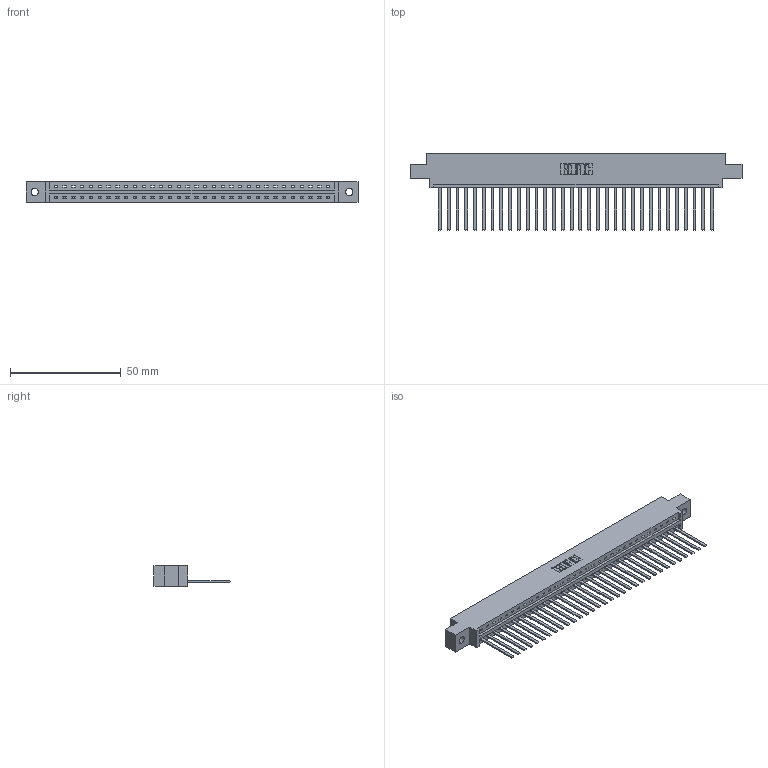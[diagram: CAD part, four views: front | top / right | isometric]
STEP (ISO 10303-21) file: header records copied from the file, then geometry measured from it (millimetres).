
FILE_DESCRIPTION (( 'STEP AP203' ), '1' );
FILE_NAME ('337-032-544-602.STEP', '2019-10-01T03:38:25', ( '' ), ( '' ), 'SwSTEP 2.0', 'SolidWorks 2016', '' );
FILE_SCHEMA (( 'CONFIG_CONTROL_DESIGN' ));
Length unit declared in the file: inch
Products named in the file (3): 337 Part_0.170 Offset - 0.128 Dia; 337-032-544-602; 345-292-001_345-293-144
Assembly tree (33 placements, depth 2):
  337-032-544-602
    337 Part_0.170 Offset - 0.128 Dia
    345-292-001_345-293-144  x32
Bounding box: 149.81 x 34.3 x 9.4 mm (x, y, z)
Volume: 15661.4 mm3; surface area: 17174 mm2
Topology: 33 solids, 33 shells, 1910 faces, 5763 edges, 3798 vertices
Faces by surface type: plane 1418, cylinder 492
Entity records: 25031 total; most frequent: CARTESIAN_POINT 4366, ORIENTED_EDGE 4334, DIRECTION 3691, EDGE_CURVE 2167, VECTOR 2043, LINE 2043, VERTEX_POINT 1442, AXIS2_PLACEMENT_3D 824
